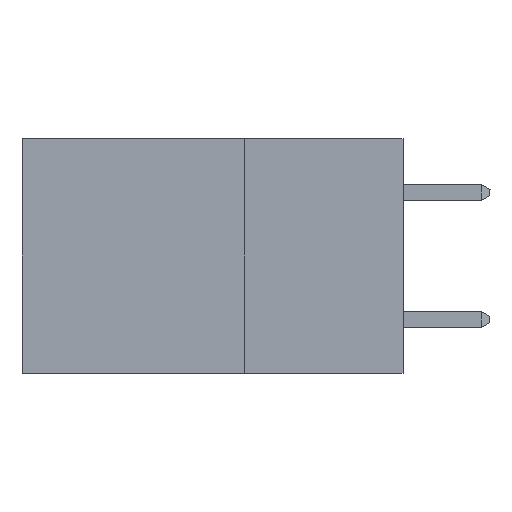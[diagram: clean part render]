
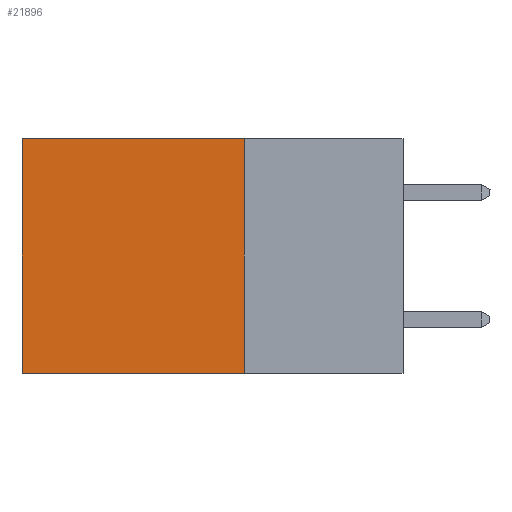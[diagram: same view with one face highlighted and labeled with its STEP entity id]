
A CAD part, left-side view. The second image highlights one B-rep face of the part: STEP entity #21896.
In plain terms, the highlighted planar face has unit normal (-1, 0, 0).
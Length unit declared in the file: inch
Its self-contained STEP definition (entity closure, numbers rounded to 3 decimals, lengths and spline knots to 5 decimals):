
#807 = CARTESIAN_POINT ( 'NONE',  ( 0.2875, 0.6, 0. ) ) ;
#834 = CARTESIAN_POINT ( 'NONE',  ( 0.2875, 0.6, -0.37 ) ) ;
#1977 = VERTEX_POINT ( 'NONE', #834 ) ;
#3531 = ORIENTED_EDGE ( 'NONE', *, *, #8577, .F. ) ;
#3966 = DIRECTION ( 'NONE',  ( 0., 1., 0. ) ) ;
#5318 = EDGE_CURVE ( 'NONE', #36502, #19488, #21083, .T. ) ;
#5866 = PLANE ( 'NONE',  #15855 ) ;
#6144 = DIRECTION ( 'NONE',  ( 0., 0., -1. ) ) ;
#6506 = CARTESIAN_POINT ( 'NONE',  ( 0.2875, 0.25, -0.37 ) ) ;
#8126 = DIRECTION ( 'NONE',  ( 0., 1., 0. ) ) ;
#8577 = EDGE_CURVE ( 'NONE', #19488, #1977, #33469, .T. ) ;
#10323 = CARTESIAN_POINT ( 'NONE',  ( 0.2875, 0.25, -0.37 ) ) ;
#14983 = ORIENTED_EDGE ( 'NONE', *, *, #33587, .T. ) ;
#15391 = CARTESIAN_POINT ( 'NONE',  ( 0.2875, 0.25, 0. ) ) ;
#15855 = AXIS2_PLACEMENT_3D ( 'NONE', #15391, #27319, #21646 ) ;
#17870 = CARTESIAN_POINT ( 'NONE',  ( 0.2875, 0.6, 0. ) ) ;
#18349 = DIRECTION ( 'NONE',  ( 0., 0., -1. ) ) ;
#18475 = LINE ( 'NONE', #17870, #21955 ) ;
#19488 = VERTEX_POINT ( 'NONE', #10323 ) ;
#19630 = CARTESIAN_POINT ( 'NONE',  ( 0.2875, 0.25, 0. ) ) ;
#19724 = VECTOR ( 'NONE', #18349, 39.37008 ) ;
#20246 = VERTEX_POINT ( 'NONE', #807 ) ;
#20285 = VECTOR ( 'NONE', #8126, 39.37008 ) ;
#20740 = EDGE_CURVE ( 'NONE', #36502, #20246, #23169, .T. ) ;
#21083 = LINE ( 'NONE', #29874, #19724 ) ;
#21646 = DIRECTION ( 'NONE',  ( 0., 0., -1. ) ) ;
#21896 = ADVANCED_FACE ( 'NONE', ( #32639 ), #5866, .F. ) ;
#21955 = VECTOR ( 'NONE', #6144, 39.37008 ) ;
#23169 = LINE ( 'NONE', #35104, #20285 ) ;
#27319 = DIRECTION ( 'NONE',  ( 1., 0., 0. ) ) ;
#29874 = CARTESIAN_POINT ( 'NONE',  ( 0.2875, 0.25, 0. ) ) ;
#32639 = FACE_OUTER_BOUND ( 'NONE', #35737, .T. ) ;
#33469 = LINE ( 'NONE', #6506, #36532 ) ;
#33587 = EDGE_CURVE ( 'NONE', #20246, #1977, #18475, .T. ) ;
#35104 = CARTESIAN_POINT ( 'NONE',  ( 0.2875, 0.25, 0. ) ) ;
#35737 = EDGE_LOOP ( 'NONE', ( #14983, #3531, #35871, #36556 ) ) ;
#35871 = ORIENTED_EDGE ( 'NONE', *, *, #5318, .F. ) ;
#36502 = VERTEX_POINT ( 'NONE', #19630 ) ;
#36532 = VECTOR ( 'NONE', #3966, 39.37008 ) ;
#36556 = ORIENTED_EDGE ( 'NONE', *, *, #20740, .T. ) ;
